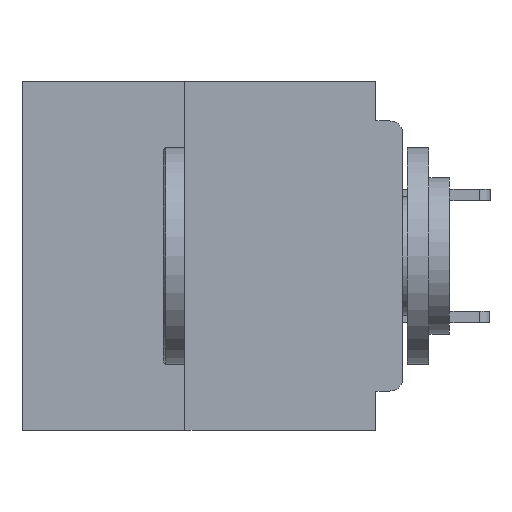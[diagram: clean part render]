
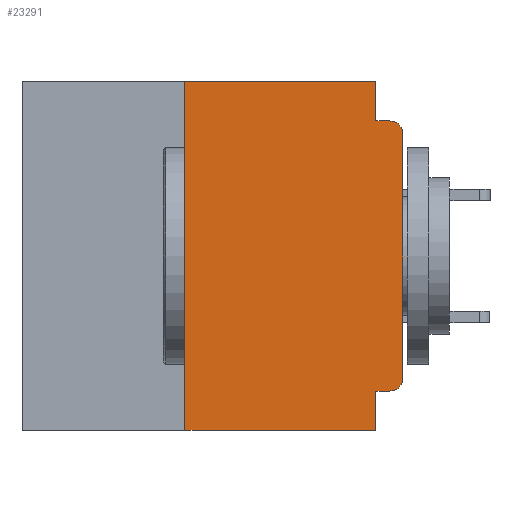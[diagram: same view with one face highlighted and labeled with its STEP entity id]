
A CAD part, left-side view. The second image highlights one B-rep face of the part: STEP entity #23291.
In plain terms, the highlighted planar face has unit normal (-1, 0, 0).
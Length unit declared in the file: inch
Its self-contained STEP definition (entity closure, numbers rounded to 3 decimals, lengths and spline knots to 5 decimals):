
#2043 = VERTEX_POINT ( 'NONE', #36853 ) ;
#2160 = EDGE_LOOP ( 'NONE', ( #10632, #20377, #4616, #23346, #7606, #33818, #17905, #34796, #12560, #20886 ) ) ;
#2528 = VECTOR ( 'NONE', #33860, 39.37008 ) ;
#2777 = VECTOR ( 'NONE', #37449, 39.37008 ) ;
#2988 = CARTESIAN_POINT ( 'NONE',  ( 0., 0., -0.34 ) ) ;
#3501 = CARTESIAN_POINT ( 'NONE',  ( 0., 0.25, -0.4 ) ) ;
#3791 = LINE ( 'NONE', #36823, #2777 ) ;
#4616 = ORIENTED_EDGE ( 'NONE', *, *, #17396, .F. ) ;
#4704 = DIRECTION ( 'NONE',  ( -1., 0., 0. ) ) ;
#4746 = EDGE_CURVE ( 'NONE', #15396, #10006, #3791, .T. ) ;
#5416 = CARTESIAN_POINT ( 'NONE',  ( 0., 0.437, 0. ) ) ;
#6155 = CARTESIAN_POINT ( 'NONE',  ( 0., 0.031, 0. ) ) ;
#6176 = LINE ( 'NONE', #38702, #12619 ) ;
#7606 = ORIENTED_EDGE ( 'NONE', *, *, #12805, .F. ) ;
#8677 = CARTESIAN_POINT ( 'NONE',  ( 0., 0.015, -0.355 ) ) ;
#9007 = VERTEX_POINT ( 'NONE', #33591 ) ;
#10006 = VERTEX_POINT ( 'NONE', #21082 ) ;
#10632 = ORIENTED_EDGE ( 'NONE', *, *, #4746, .T. ) ;
#10765 = AXIS2_PLACEMENT_3D ( 'NONE', #23583, #4704, #26831 ) ;
#11242 = EDGE_CURVE ( 'NONE', #10006, #35703, #25069, .T. ) ;
#12560 = ORIENTED_EDGE ( 'NONE', *, *, #14764, .F. ) ;
#12619 = VECTOR ( 'NONE', #13393, 39.37008 ) ;
#12805 = EDGE_CURVE ( 'NONE', #9007, #28719, #12959, .T. ) ;
#12878 = LINE ( 'NONE', #6155, #20225 ) ;
#12959 = LINE ( 'NONE', #14615, #27792 ) ;
#12999 = EDGE_CURVE ( 'NONE', #28071, #9007, #14383, .T. ) ;
#13393 = DIRECTION ( 'NONE',  ( 0., -1., 0. ) ) ;
#13420 = VECTOR ( 'NONE', #31373, 39.37008 ) ;
#13699 = EDGE_CURVE ( 'NONE', #28719, #21829, #12878, .T. ) ;
#14383 = LINE ( 'NONE', #28192, #13420 ) ;
#14615 = CARTESIAN_POINT ( 'NONE',  ( 0., 0.437, 0. ) ) ;
#14764 = EDGE_CURVE ( 'NONE', #27861, #2043, #31089, .T. ) ;
#14907 = DIRECTION ( 'NONE',  ( 1., 0., 0. ) ) ;
#15396 = VERTEX_POINT ( 'NONE', #2988 ) ;
#15650 = DIRECTION ( 'NONE',  ( 0., 0., -1. ) ) ;
#16656 = DIRECTION ( 'NONE',  ( -1., 0., 0. ) ) ;
#17396 = EDGE_CURVE ( 'NONE', #21829, #35703, #6176, .T. ) ;
#17905 = ORIENTED_EDGE ( 'NONE', *, *, #37111, .T. ) ;
#18961 = FACE_OUTER_BOUND ( 'NONE', #2160, .T. ) ;
#20225 = VECTOR ( 'NONE', #15650, 39.37008 ) ;
#20377 = ORIENTED_EDGE ( 'NONE', *, *, #11242, .T. ) ;
#20689 = CARTESIAN_POINT ( 'NONE',  ( 0., 0.031, -0.4 ) ) ;
#20886 = ORIENTED_EDGE ( 'NONE', *, *, #40785, .T. ) ;
#20938 = DIRECTION ( 'NONE',  ( 0., -1., 0. ) ) ;
#21082 = CARTESIAN_POINT ( 'NONE',  ( 0., 0., -0.06 ) ) ;
#21606 = VECTOR ( 'NONE', #33729, 39.37008 ) ;
#21829 = VERTEX_POINT ( 'NONE', #23564 ) ;
#23291 = ADVANCED_FACE ( 'NONE', ( #18961 ), #33904, .F. ) ;
#23346 = ORIENTED_EDGE ( 'NONE', *, *, #13699, .F. ) ;
#23564 = CARTESIAN_POINT ( 'NONE',  ( 0., 0.031, -0.045 ) ) ;
#23583 = CARTESIAN_POINT ( 'NONE',  ( 0., 0.015, -0.06 ) ) ;
#24793 = AXIS2_PLACEMENT_3D ( 'NONE', #35654, #16656, #38851 ) ;
#25069 = CIRCLE ( 'NONE', #10765, 0.015 ) ;
#26363 = AXIS2_PLACEMENT_3D ( 'NONE', #5416, #14907, #37079 ) ;
#26630 = CARTESIAN_POINT ( 'NONE',  ( 0., 0.015, -0.045 ) ) ;
#26831 = DIRECTION ( 'NONE',  ( 0., 0., -1. ) ) ;
#27792 = VECTOR ( 'NONE', #20938, 39.37008 ) ;
#27817 = LINE ( 'NONE', #30686, #2528 ) ;
#27861 = VERTEX_POINT ( 'NONE', #8677 ) ;
#28071 = VERTEX_POINT ( 'NONE', #3501 ) ;
#28192 = CARTESIAN_POINT ( 'NONE',  ( 0., 0.25, -0.4 ) ) ;
#28719 = VERTEX_POINT ( 'NONE', #38052 ) ;
#29573 = CARTESIAN_POINT ( 'NONE',  ( 0., 0.031, -0.4 ) ) ;
#30372 = LINE ( 'NONE', #29573, #37782 ) ;
#30587 = EDGE_CURVE ( 'NONE', #2043, #40438, #30372, .T. ) ;
#30686 = CARTESIAN_POINT ( 'NONE',  ( 0., 0.437, -0.4 ) ) ;
#31089 = LINE ( 'NONE', #33584, #21606 ) ;
#31373 = DIRECTION ( 'NONE',  ( 0., 0., 1. ) ) ;
#32743 = DIRECTION ( 'NONE',  ( 0., 0., -1. ) ) ;
#33584 = CARTESIAN_POINT ( 'NONE',  ( 0., 0., -0.355 ) ) ;
#33591 = CARTESIAN_POINT ( 'NONE',  ( 0., 0.25, 0. ) ) ;
#33729 = DIRECTION ( 'NONE',  ( 0., 1., 0. ) ) ;
#33818 = ORIENTED_EDGE ( 'NONE', *, *, #12999, .F. ) ;
#33860 = DIRECTION ( 'NONE',  ( 0., -1., 0. ) ) ;
#33904 = PLANE ( 'NONE',  #26363 ) ;
#34796 = ORIENTED_EDGE ( 'NONE', *, *, #30587, .F. ) ;
#35654 = CARTESIAN_POINT ( 'NONE',  ( 0., 0.015, -0.34 ) ) ;
#35703 = VERTEX_POINT ( 'NONE', #26630 ) ;
#36823 = CARTESIAN_POINT ( 'NONE',  ( 0., 0., 0. ) ) ;
#36853 = CARTESIAN_POINT ( 'NONE',  ( 0., 0.031, -0.355 ) ) ;
#37079 = DIRECTION ( 'NONE',  ( 0., 0., -1. ) ) ;
#37111 = EDGE_CURVE ( 'NONE', #28071, #40438, #27817, .T. ) ;
#37449 = DIRECTION ( 'NONE',  ( 0., 0., 1. ) ) ;
#37782 = VECTOR ( 'NONE', #32743, 39.37008 ) ;
#38052 = CARTESIAN_POINT ( 'NONE',  ( 0., 0.031, 0. ) ) ;
#38702 = CARTESIAN_POINT ( 'NONE',  ( 0., 0., -0.045 ) ) ;
#38851 = DIRECTION ( 'NONE',  ( 0., 0., -1. ) ) ;
#38905 = CIRCLE ( 'NONE', #24793, 0.015 ) ;
#40438 = VERTEX_POINT ( 'NONE', #20689 ) ;
#40785 = EDGE_CURVE ( 'NONE', #27861, #15396, #38905, .T. ) ;
